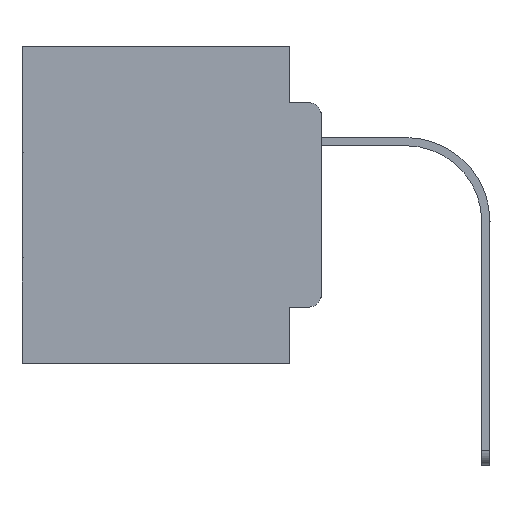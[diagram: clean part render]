
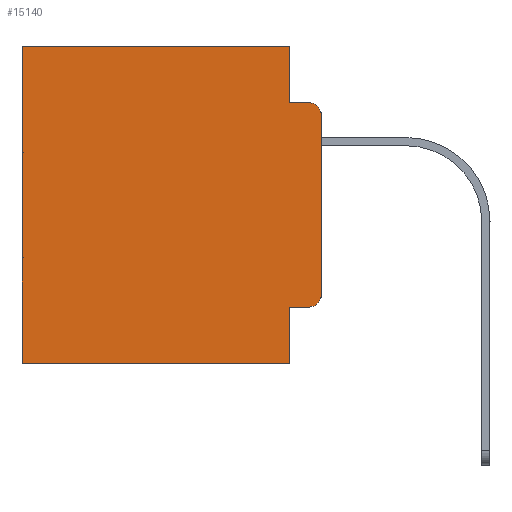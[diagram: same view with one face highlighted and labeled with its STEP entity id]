
A CAD part, left-side view. The second image highlights one B-rep face of the part: STEP entity #15140.
In plain terms, the highlighted planar face has unit normal (-1, 0, 0).
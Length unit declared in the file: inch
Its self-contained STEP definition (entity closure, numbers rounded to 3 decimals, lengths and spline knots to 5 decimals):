
#123 = CARTESIAN_POINT ( 'NONE',  ( 0.298, 0.051, -0.4115 ) ) ;
#132 = VERTEX_POINT ( 'NONE', #23352 ) ;
#839 = ORIENTED_EDGE ( 'NONE', *, *, #20711, .F. ) ;
#995 = ORIENTED_EDGE ( 'NONE', *, *, #15799, .T. ) ;
#1142 = ORIENTED_EDGE ( 'NONE', *, *, #13174, .T. ) ;
#1471 = VERTEX_POINT ( 'NONE', #4201 ) ;
#1802 = CARTESIAN_POINT ( 'NONE',  ( 0.298, 0.473, -0.5 ) ) ;
#1834 = CARTESIAN_POINT ( 'NONE',  ( 0.298, 0., -0.3915 ) ) ;
#2205 = LINE ( 'NONE', #123, #17941 ) ;
#2222 = ORIENTED_EDGE ( 'NONE', *, *, #11303, .T. ) ;
#3717 = CIRCLE ( 'NONE', #13655, 0.02 ) ;
#4084 = CARTESIAN_POINT ( 'NONE',  ( 0.298, 0.473, 0. ) ) ;
#4142 = VERTEX_POINT ( 'NONE', #1802 ) ;
#4201 = CARTESIAN_POINT ( 'NONE',  ( 0.298, 0.051, -0.5 ) ) ;
#4818 = VECTOR ( 'NONE', #8014, 39.37008 ) ;
#5419 = EDGE_CURVE ( 'NONE', #28156, #18113, #15717, .T. ) ;
#6244 = AXIS2_PLACEMENT_3D ( 'NONE', #16211, #11196, #9112 ) ;
#6666 = ORIENTED_EDGE ( 'NONE', *, *, #18972, .F. ) ;
#6959 = EDGE_CURVE ( 'NONE', #12964, #22978, #28976, .T. ) ;
#8014 = DIRECTION ( 'NONE',  ( 0., -1., 0. ) ) ;
#8034 = DIRECTION ( 'NONE',  ( 0., 1., 0. ) ) ;
#8157 = DIRECTION ( 'NONE',  ( 0., 0., -1. ) ) ;
#9085 = CARTESIAN_POINT ( 'NONE',  ( 0.298, 0.02, -0.0885 ) ) ;
#9101 = VECTOR ( 'NONE', #11217, 39.37008 ) ;
#9112 = DIRECTION ( 'NONE',  ( 0., 0., -1. ) ) ;
#10656 = DIRECTION ( 'NONE',  ( 0., 0., -1. ) ) ;
#11196 = DIRECTION ( 'NONE',  ( -1., 0., 0. ) ) ;
#11217 = DIRECTION ( 'NONE',  ( 0., 0., -1. ) ) ;
#11238 = DIRECTION ( 'NONE',  ( 0., -1., 0. ) ) ;
#11303 = EDGE_CURVE ( 'NONE', #132, #12317, #2205, .T. ) ;
#11515 = AXIS2_PLACEMENT_3D ( 'NONE', #23099, #25308, #22953 ) ;
#12300 = EDGE_CURVE ( 'NONE', #12317, #18113, #3717, .T. ) ;
#12317 = VERTEX_POINT ( 'NONE', #15982 ) ;
#12336 = LINE ( 'NONE', #25773, #24327 ) ;
#12964 = VERTEX_POINT ( 'NONE', #14163 ) ;
#13026 = EDGE_LOOP ( 'NONE', ( #16690, #995, #27278, #28653, #23001, #1142, #839, #6666, #2222, #27629 ) ) ;
#13174 = EDGE_CURVE ( 'NONE', #22978, #4142, #24328, .T. ) ;
#13655 = AXIS2_PLACEMENT_3D ( 'NONE', #28402, #15121, #8157 ) ;
#14163 = CARTESIAN_POINT ( 'NONE',  ( 0.298, 0.051, 0. ) ) ;
#14745 = VERTEX_POINT ( 'NONE', #21060 ) ;
#14755 = VECTOR ( 'NONE', #22106, 39.37008 ) ;
#15121 = DIRECTION ( 'NONE',  ( -1., 0., 0. ) ) ;
#15140 = ADVANCED_FACE ( 'NONE', ( #27830 ), #25455, .F. ) ;
#15717 = LINE ( 'NONE', #24713, #17765 ) ;
#15799 = EDGE_CURVE ( 'NONE', #28156, #20474, #27946, .T. ) ;
#15982 = CARTESIAN_POINT ( 'NONE',  ( 0.298, 0.02, -0.4115 ) ) ;
#16211 = CARTESIAN_POINT ( 'NONE',  ( 0.298, 0.02, -0.1085 ) ) ;
#16279 = EDGE_CURVE ( 'NONE', #14745, #20474, #18963, .T. ) ;
#16690 = ORIENTED_EDGE ( 'NONE', *, *, #5419, .F. ) ;
#17765 = VECTOR ( 'NONE', #22496, 39.37008 ) ;
#17893 = EDGE_CURVE ( 'NONE', #12964, #14745, #24650, .T. ) ;
#17941 = VECTOR ( 'NONE', #11238, 39.37008 ) ;
#18113 = VERTEX_POINT ( 'NONE', #1834 ) ;
#18963 = LINE ( 'NONE', #28253, #4818 ) ;
#18972 = EDGE_CURVE ( 'NONE', #132, #1471, #24367, .T. ) ;
#20474 = VERTEX_POINT ( 'NONE', #9085 ) ;
#20711 = EDGE_CURVE ( 'NONE', #1471, #4142, #12336, .T. ) ;
#21060 = CARTESIAN_POINT ( 'NONE',  ( 0.298, 0.051, -0.0885 ) ) ;
#22106 = DIRECTION ( 'NONE',  ( 0., 0., -1. ) ) ;
#22147 = CARTESIAN_POINT ( 'NONE',  ( 0.298, 0.051, 0. ) ) ;
#22243 = CARTESIAN_POINT ( 'NONE',  ( 0.298, 0., -0.1085 ) ) ;
#22496 = DIRECTION ( 'NONE',  ( 0., 0., -1. ) ) ;
#22582 = CARTESIAN_POINT ( 'NONE',  ( 0.298, 0.051, 0. ) ) ;
#22953 = DIRECTION ( 'NONE',  ( 0., 0., -1. ) ) ;
#22978 = VERTEX_POINT ( 'NONE', #24203 ) ;
#23001 = ORIENTED_EDGE ( 'NONE', *, *, #6959, .T. ) ;
#23099 = CARTESIAN_POINT ( 'NONE',  ( 0.298, 0., 0. ) ) ;
#23352 = CARTESIAN_POINT ( 'NONE',  ( 0.298, 0.051, -0.4115 ) ) ;
#24203 = CARTESIAN_POINT ( 'NONE',  ( 0.298, 0.473, 0. ) ) ;
#24327 = VECTOR ( 'NONE', #8034, 39.37008 ) ;
#24328 = LINE ( 'NONE', #4084, #14755 ) ;
#24367 = LINE ( 'NONE', #22147, #25165 ) ;
#24650 = LINE ( 'NONE', #22582, #9101 ) ;
#24713 = CARTESIAN_POINT ( 'NONE',  ( 0.298, 0., 0. ) ) ;
#24826 = CARTESIAN_POINT ( 'NONE',  ( 0.298, 0., 0. ) ) ;
#25165 = VECTOR ( 'NONE', #10656, 39.37008 ) ;
#25308 = DIRECTION ( 'NONE',  ( 1., 0., 0. ) ) ;
#25455 = PLANE ( 'NONE',  #11515 ) ;
#25773 = CARTESIAN_POINT ( 'NONE',  ( 0.298, 0., -0.5 ) ) ;
#26619 = DIRECTION ( 'NONE',  ( 0., 1., 0. ) ) ;
#26695 = VECTOR ( 'NONE', #26619, 39.37008 ) ;
#27278 = ORIENTED_EDGE ( 'NONE', *, *, #16279, .F. ) ;
#27629 = ORIENTED_EDGE ( 'NONE', *, *, #12300, .T. ) ;
#27830 = FACE_OUTER_BOUND ( 'NONE', #13026, .T. ) ;
#27946 = CIRCLE ( 'NONE', #6244, 0.02 ) ;
#28156 = VERTEX_POINT ( 'NONE', #22243 ) ;
#28253 = CARTESIAN_POINT ( 'NONE',  ( 0.298, 0.051, -0.0885 ) ) ;
#28402 = CARTESIAN_POINT ( 'NONE',  ( 0.298, 0.02, -0.3915 ) ) ;
#28653 = ORIENTED_EDGE ( 'NONE', *, *, #17893, .F. ) ;
#28976 = LINE ( 'NONE', #24826, #26695 ) ;
